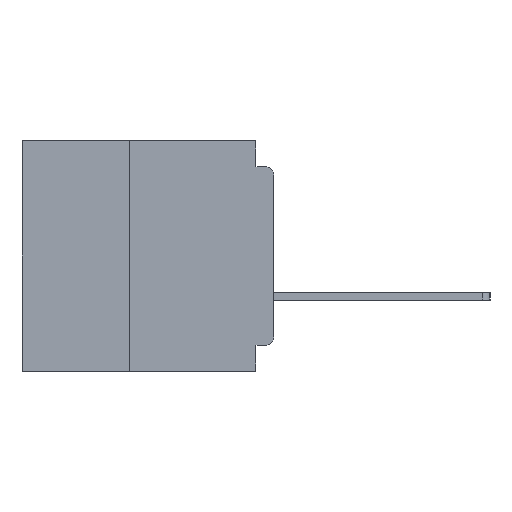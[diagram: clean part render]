
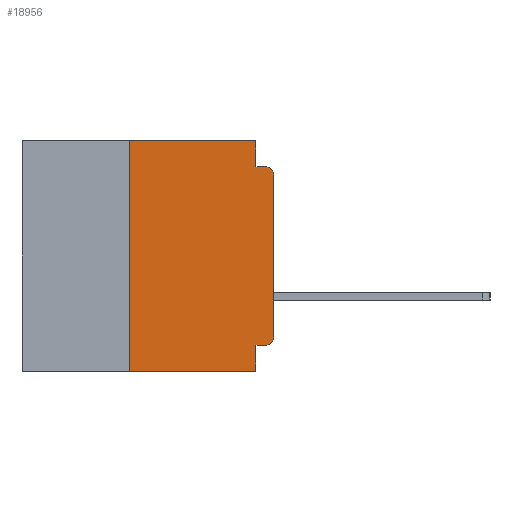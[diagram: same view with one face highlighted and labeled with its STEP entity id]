
A CAD part, left-side view. The second image highlights one B-rep face of the part: STEP entity #18956.
In plain terms, the highlighted planar face has unit normal (-1, 0, 0).
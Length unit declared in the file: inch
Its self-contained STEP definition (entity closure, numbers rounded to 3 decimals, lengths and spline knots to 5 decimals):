
#1113 = DIRECTION ( 'NONE',  ( 0., 0., 1. ) ) ;
#1244 = CARTESIAN_POINT ( 'NONE',  ( 0., 0.25, -0.4 ) ) ;
#1442 = LINE ( 'NONE', #15280, #33087 ) ;
#2471 = AXIS2_PLACEMENT_3D ( 'NONE', #4680, #7666, #28422 ) ;
#3057 = EDGE_CURVE ( 'NONE', #11132, #29523, #29287, .T. ) ;
#3201 = ORIENTED_EDGE ( 'NONE', *, *, #29104, .T. ) ;
#4680 = CARTESIAN_POINT ( 'NONE',  ( 0., 0.437, 0. ) ) ;
#5095 = DIRECTION ( 'NONE',  ( 0., 1., 0. ) ) ;
#5106 = AXIS2_PLACEMENT_3D ( 'NONE', #5857, #26602, #8858 ) ;
#5189 = DIRECTION ( 'NONE',  ( 0., -1., 0. ) ) ;
#5223 = LINE ( 'NONE', #34802, #27962 ) ;
#5291 = VECTOR ( 'NONE', #5189, 39.37008 ) ;
#5799 = EDGE_CURVE ( 'NONE', #28942, #11132, #6870, .T. ) ;
#5857 = CARTESIAN_POINT ( 'NONE',  ( 0., 0.015, -0.34 ) ) ;
#6870 = CIRCLE ( 'NONE', #5106, 0.015 ) ;
#6996 = ORIENTED_EDGE ( 'NONE', *, *, #7793, .F. ) ;
#7666 = DIRECTION ( 'NONE',  ( 1., 0., 0. ) ) ;
#7793 = EDGE_CURVE ( 'NONE', #37298, #27720, #21070, .T. ) ;
#8130 = CARTESIAN_POINT ( 'NONE',  ( 0., 0.25, -0.4 ) ) ;
#8185 = CARTESIAN_POINT ( 'NONE',  ( 0., 0., -0.045 ) ) ;
#8586 = CIRCLE ( 'NONE', #11676, 0.015 ) ;
#8858 = DIRECTION ( 'NONE',  ( 0., 0., -1. ) ) ;
#9427 = CARTESIAN_POINT ( 'NONE',  ( 0., 0.031, -0.045 ) ) ;
#9742 = ORIENTED_EDGE ( 'NONE', *, *, #26297, .F. ) ;
#10455 = LINE ( 'NONE', #16807, #25312 ) ;
#11132 = VERTEX_POINT ( 'NONE', #32166 ) ;
#11623 = VERTEX_POINT ( 'NONE', #8130 ) ;
#11676 = AXIS2_PLACEMENT_3D ( 'NONE', #31996, #14171, #34964 ) ;
#13045 = ORIENTED_EDGE ( 'NONE', *, *, #5799, .T. ) ;
#13513 = CARTESIAN_POINT ( 'NONE',  ( 0., 0.015, -0.355 ) ) ;
#14164 = ORIENTED_EDGE ( 'NONE', *, *, #3057, .T. ) ;
#14171 = DIRECTION ( 'NONE',  ( -1., 0., 0. ) ) ;
#14221 = EDGE_CURVE ( 'NONE', #28942, #34424, #5223, .T. ) ;
#14274 = DIRECTION ( 'NONE',  ( 0., -1., 0. ) ) ;
#14378 = VECTOR ( 'NONE', #31709, 39.37008 ) ;
#14964 = EDGE_CURVE ( 'NONE', #18019, #37298, #1442, .T. ) ;
#15280 = CARTESIAN_POINT ( 'NONE',  ( 0., 0.031, 0. ) ) ;
#15459 = CARTESIAN_POINT ( 'NONE',  ( 0., 0.031, -0.355 ) ) ;
#16807 = CARTESIAN_POINT ( 'NONE',  ( 0., 0.031, -0.4 ) ) ;
#18019 = VERTEX_POINT ( 'NONE', #26134 ) ;
#18460 = EDGE_CURVE ( 'NONE', #33763, #18019, #22346, .T. ) ;
#18956 = ADVANCED_FACE ( 'NONE', ( #20457 ), #22438, .F. ) ;
#19132 = VERTEX_POINT ( 'NONE', #32182 ) ;
#19228 = CARTESIAN_POINT ( 'NONE',  ( 0., 0., -0.06 ) ) ;
#19344 = LINE ( 'NONE', #1244, #27246 ) ;
#19606 = ORIENTED_EDGE ( 'NONE', *, *, #14221, .F. ) ;
#19798 = DIRECTION ( 'NONE',  ( 0., 0., -1. ) ) ;
#20457 = FACE_OUTER_BOUND ( 'NONE', #33666, .T. ) ;
#21057 = ORIENTED_EDGE ( 'NONE', *, *, #36165, .T. ) ;
#21070 = LINE ( 'NONE', #8185, #5291 ) ;
#22346 = LINE ( 'NONE', #29119, #37140 ) ;
#22438 = PLANE ( 'NONE',  #2471 ) ;
#24203 = CARTESIAN_POINT ( 'NONE',  ( 0., 0.25, 0. ) ) ;
#24395 = ORIENTED_EDGE ( 'NONE', *, *, #14964, .F. ) ;
#25312 = VECTOR ( 'NONE', #19798, 39.37008 ) ;
#26134 = CARTESIAN_POINT ( 'NONE',  ( 0., 0.031, 0. ) ) ;
#26297 = EDGE_CURVE ( 'NONE', #34424, #19132, #10455, .T. ) ;
#26602 = DIRECTION ( 'NONE',  ( -1., 0., 0. ) ) ;
#27246 = VECTOR ( 'NONE', #1113, 39.37008 ) ;
#27720 = VERTEX_POINT ( 'NONE', #31170 ) ;
#27962 = VECTOR ( 'NONE', #5095, 39.37008 ) ;
#28182 = EDGE_CURVE ( 'NONE', #11623, #33763, #19344, .T. ) ;
#28422 = DIRECTION ( 'NONE',  ( 0., 0., -1. ) ) ;
#28600 = ORIENTED_EDGE ( 'NONE', *, *, #28182, .F. ) ;
#28942 = VERTEX_POINT ( 'NONE', #13513 ) ;
#29104 = EDGE_CURVE ( 'NONE', #29523, #27720, #8586, .T. ) ;
#29119 = CARTESIAN_POINT ( 'NONE',  ( 0., 0.437, 0. ) ) ;
#29287 = LINE ( 'NONE', #31447, #14378 ) ;
#29523 = VERTEX_POINT ( 'NONE', #19228 ) ;
#30554 = CARTESIAN_POINT ( 'NONE',  ( 0., 0.437, -0.4 ) ) ;
#30750 = LINE ( 'NONE', #30554, #37613 ) ;
#31170 = CARTESIAN_POINT ( 'NONE',  ( 0., 0.015, -0.045 ) ) ;
#31447 = CARTESIAN_POINT ( 'NONE',  ( 0., 0., 0. ) ) ;
#31709 = DIRECTION ( 'NONE',  ( 0., 0., 1. ) ) ;
#31996 = CARTESIAN_POINT ( 'NONE',  ( 0., 0.015, -0.06 ) ) ;
#32166 = CARTESIAN_POINT ( 'NONE',  ( 0., 0., -0.34 ) ) ;
#32182 = CARTESIAN_POINT ( 'NONE',  ( 0., 0.031, -0.4 ) ) ;
#33010 = ORIENTED_EDGE ( 'NONE', *, *, #18460, .F. ) ;
#33087 = VECTOR ( 'NONE', #36039, 39.37008 ) ;
#33527 = DIRECTION ( 'NONE',  ( 0., -1., 0. ) ) ;
#33666 = EDGE_LOOP ( 'NONE', ( #14164, #3201, #6996, #24395, #33010, #28600, #21057, #9742, #19606, #13045 ) ) ;
#33763 = VERTEX_POINT ( 'NONE', #24203 ) ;
#34424 = VERTEX_POINT ( 'NONE', #15459 ) ;
#34802 = CARTESIAN_POINT ( 'NONE',  ( 0., 0., -0.355 ) ) ;
#34964 = DIRECTION ( 'NONE',  ( 0., 0., -1. ) ) ;
#36039 = DIRECTION ( 'NONE',  ( 0., 0., -1. ) ) ;
#36165 = EDGE_CURVE ( 'NONE', #11623, #19132, #30750, .T. ) ;
#37140 = VECTOR ( 'NONE', #14274, 39.37008 ) ;
#37298 = VERTEX_POINT ( 'NONE', #9427 ) ;
#37613 = VECTOR ( 'NONE', #33527, 39.37008 ) ;
